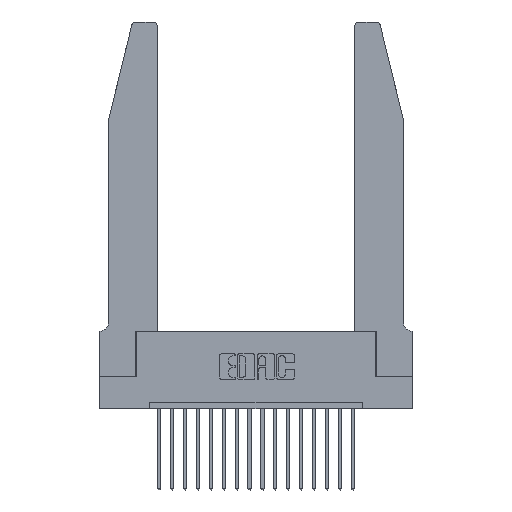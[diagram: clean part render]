
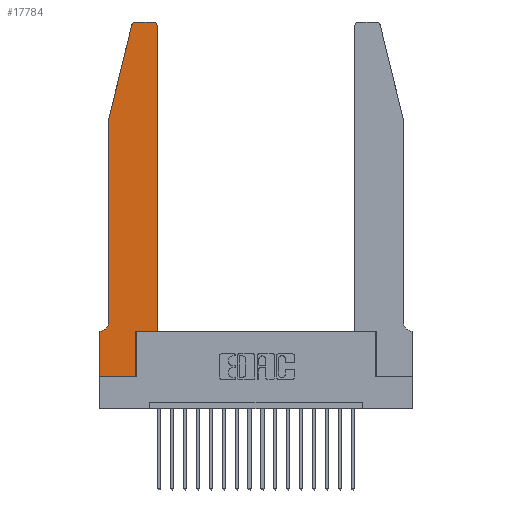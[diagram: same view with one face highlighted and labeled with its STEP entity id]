
A CAD part, top view. The second image highlights one B-rep face of the part: STEP entity #17784.
In plain terms, the highlighted planar face has unit normal (0, 0, 1).
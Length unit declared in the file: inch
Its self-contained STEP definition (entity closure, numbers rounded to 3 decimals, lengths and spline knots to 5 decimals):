
#45 = CIRCLE ( 'NONE', #5649, 0.07 ) ;
#159 = ORIENTED_EDGE ( 'NONE', *, *, #10974, .T. ) ;
#170 = VECTOR ( 'NONE', #8607, 39.37008 ) ;
#180 = ORIENTED_EDGE ( 'NONE', *, *, #13950, .T. ) ;
#245 = CIRCLE ( 'NONE', #19819, 0.03 ) ;
#307 = VECTOR ( 'NONE', #19889, 39.37008 ) ;
#816 = LINE ( 'NONE', #15132, #307 ) ;
#843 = CARTESIAN_POINT ( 'NONE',  ( 0., 0., 0.37 ) ) ;
#1480 = CARTESIAN_POINT ( 'NONE',  ( 0., 0.35, 0.37 ) ) ;
#1695 = DIRECTION ( 'NONE',  ( 1., 0., 0. ) ) ;
#1891 = EDGE_CURVE ( 'NONE', #12858, #2792, #12460, .T. ) ;
#2074 = ORIENTED_EDGE ( 'NONE', *, *, #19408, .T. ) ;
#2139 = ORIENTED_EDGE ( 'NONE', *, *, #1891, .T. ) ;
#2157 = VERTEX_POINT ( 'NONE', #17885 ) ;
#2242 = CARTESIAN_POINT ( 'NONE',  ( 0.0755, 0.42, 0.37 ) ) ;
#2270 = ORIENTED_EDGE ( 'NONE', *, *, #5480, .T. ) ;
#2278 = ORIENTED_EDGE ( 'NONE', *, *, #17199, .T. ) ;
#2341 = VERTEX_POINT ( 'NONE', #13938 ) ;
#2727 = VERTEX_POINT ( 'NONE', #8370 ) ;
#2756 = DIRECTION ( 'NONE',  ( 1., 0., 0. ) ) ;
#2769 = VERTEX_POINT ( 'NONE', #18088 ) ;
#2771 = VERTEX_POINT ( 'NONE', #8446 ) ;
#2792 = VERTEX_POINT ( 'NONE', #16397 ) ;
#3001 = CARTESIAN_POINT ( 'NONE',  ( 0.4505, 0.35, 0.37 ) ) ;
#3121 = CARTESIAN_POINT ( 'NONE',  ( 0.4205, 2.72, 0.37 ) ) ;
#3135 = ORIENTED_EDGE ( 'NONE', *, *, #17731, .T. ) ;
#3656 = EDGE_CURVE ( 'NONE', #15645, #12858, #9179, .T. ) ;
#3837 = DIRECTION ( 'NONE',  ( 1., 0., 0. ) ) ;
#4051 = VECTOR ( 'NONE', #12001, 39.37008 ) ;
#4215 = VECTOR ( 'NONE', #16159, 39.37008 ) ;
#4398 = EDGE_CURVE ( 'NONE', #2341, #15154, #12325, .T. ) ;
#4415 = DIRECTION ( 'NONE',  ( 0., 1., 0. ) ) ;
#4730 = CARTESIAN_POINT ( 'NONE',  ( 0., 0.35, 0.37 ) ) ;
#5480 = EDGE_CURVE ( 'NONE', #12224, #2771, #11797, .T. ) ;
#5498 = ORIENTED_EDGE ( 'NONE', *, *, #3656, .T. ) ;
#5649 = AXIS2_PLACEMENT_3D ( 'NONE', #6503, #19062, #11214 ) ;
#5701 = DIRECTION ( 'NONE',  ( 0., -1., 0. ) ) ;
#5798 = CARTESIAN_POINT ( 'NONE',  ( 0.0755, 0.35, 0.37 ) ) ;
#5837 = DIRECTION ( 'NONE',  ( 0., -1., 0. ) ) ;
#6100 = CARTESIAN_POINT ( 'NONE',  ( 0.0755, 2., 0.37 ) ) ;
#6224 = LINE ( 'NONE', #5798, #4051 ) ;
#6336 = DIRECTION ( 'NONE',  ( 0., 0., 1. ) ) ;
#6437 = FACE_OUTER_BOUND ( 'NONE', #14455, .T. ) ;
#6503 = CARTESIAN_POINT ( 'NONE',  ( 0.0055, 0.42, 0.37 ) ) ;
#6614 = CIRCLE ( 'NONE', #17047, 0.03 ) ;
#6685 = ORIENTED_EDGE ( 'NONE', *, *, #12951, .T. ) ;
#7350 = VECTOR ( 'NONE', #5837, 39.37008 ) ;
#7901 = CARTESIAN_POINT ( 'NONE',  ( 0.2865, 0.35, 0.37 ) ) ;
#8370 = CARTESIAN_POINT ( 'NONE',  ( 0.284, 2.75, 0.37 ) ) ;
#8446 = CARTESIAN_POINT ( 'NONE',  ( 0.4505, 0.35, 0.37 ) ) ;
#8607 = DIRECTION ( 'NONE',  ( -1., 0., 0. ) ) ;
#8786 = CARTESIAN_POINT ( 'NONE',  ( 0.4505, 2.72, 0.37 ) ) ;
#8937 = CARTESIAN_POINT ( 'NONE',  ( 0.4505, 0.35, 0.37 ) ) ;
#9179 = LINE ( 'NONE', #18357, #11635 ) ;
#9505 = CARTESIAN_POINT ( 'NONE',  ( 0.0755, 2., 0.37 ) ) ;
#9609 = VERTEX_POINT ( 'NONE', #8786 ) ;
#10771 = VECTOR ( 'NONE', #3837, 39.37008 ) ;
#10910 = LINE ( 'NONE', #8937, #13366 ) ;
#10974 = EDGE_CURVE ( 'NONE', #20110, #2769, #45, .T. ) ;
#11050 = CARTESIAN_POINT ( 'NONE',  ( 0.284, 2.72, 0.37 ) ) ;
#11214 = DIRECTION ( 'NONE',  ( -1., 0., 0. ) ) ;
#11635 = VECTOR ( 'NONE', #5701, 39.37008 ) ;
#11797 = LINE ( 'NONE', #3001, #4215 ) ;
#11861 = AXIS2_PLACEMENT_3D ( 'NONE', #4730, #12433, #2756 ) ;
#11885 = CARTESIAN_POINT ( 'NONE',  ( 0., 0., 0.37 ) ) ;
#12001 = DIRECTION ( 'NONE',  ( -1., 0., 0. ) ) ;
#12224 = VERTEX_POINT ( 'NONE', #7901 ) ;
#12325 = LINE ( 'NONE', #6100, #14036 ) ;
#12366 = DIRECTION ( 'NONE',  ( -0.239, -0.971, 0. ) ) ;
#12433 = DIRECTION ( 'NONE',  ( 0., 0., 1. ) ) ;
#12460 = LINE ( 'NONE', #11885, #10771 ) ;
#12858 = VERTEX_POINT ( 'NONE', #843 ) ;
#12951 = EDGE_CURVE ( 'NONE', #15154, #20110, #13453, .T. ) ;
#13366 = VECTOR ( 'NONE', #4415, 39.37008 ) ;
#13453 = LINE ( 'NONE', #19884, #7350 ) ;
#13659 = ORIENTED_EDGE ( 'NONE', *, *, #19331, .T. ) ;
#13938 = CARTESIAN_POINT ( 'NONE',  ( 0.25487, 2.72718, 0.37 ) ) ;
#13950 = EDGE_CURVE ( 'NONE', #2157, #2727, #17122, .T. ) ;
#14036 = VECTOR ( 'NONE', #12366, 39.37008 ) ;
#14455 = EDGE_LOOP ( 'NONE', ( #180, #13659, #19462, #6685, #159, #2278, #5498, #2139, #3135, #2270, #19926, #2074 ) ) ;
#14808 = CARTESIAN_POINT ( 'NONE',  ( 0.2605, 2.75, 0.37 ) ) ;
#15132 = CARTESIAN_POINT ( 'NONE',  ( 0.2865, 0.35, 0.37 ) ) ;
#15154 = VERTEX_POINT ( 'NONE', #9505 ) ;
#15645 = VERTEX_POINT ( 'NONE', #1480 ) ;
#15932 = PLANE ( 'NONE',  #11861 ) ;
#16128 = EDGE_CURVE ( 'NONE', #2771, #9609, #10910, .T. ) ;
#16159 = DIRECTION ( 'NONE',  ( 1., 0., 0. ) ) ;
#16397 = CARTESIAN_POINT ( 'NONE',  ( 0.2865, 0., 0.37 ) ) ;
#17047 = AXIS2_PLACEMENT_3D ( 'NONE', #11050, #6336, #1695 ) ;
#17122 = LINE ( 'NONE', #14808, #170 ) ;
#17199 = EDGE_CURVE ( 'NONE', #2769, #15645, #6224, .T. ) ;
#17393 = DIRECTION ( 'NONE',  ( 1., 0., 0. ) ) ;
#17731 = EDGE_CURVE ( 'NONE', #2792, #12224, #816, .T. ) ;
#17784 = ADVANCED_FACE ( 'NONE', ( #6437 ), #15932, .T. ) ;
#17885 = CARTESIAN_POINT ( 'NONE',  ( 0.4205, 2.75, 0.37 ) ) ;
#18088 = CARTESIAN_POINT ( 'NONE',  ( 0.0055, 0.35, 0.37 ) ) ;
#18357 = CARTESIAN_POINT ( 'NONE',  ( 0., 0., 0.37 ) ) ;
#18752 = DIRECTION ( 'NONE',  ( 0., 0., 1. ) ) ;
#19062 = DIRECTION ( 'NONE',  ( 0., 0., -1. ) ) ;
#19331 = EDGE_CURVE ( 'NONE', #2727, #2341, #6614, .T. ) ;
#19408 = EDGE_CURVE ( 'NONE', #9609, #2157, #245, .T. ) ;
#19462 = ORIENTED_EDGE ( 'NONE', *, *, #4398, .T. ) ;
#19819 = AXIS2_PLACEMENT_3D ( 'NONE', #3121, #18752, #17393 ) ;
#19884 = CARTESIAN_POINT ( 'NONE',  ( 0.0755, 2., 0.37 ) ) ;
#19889 = DIRECTION ( 'NONE',  ( 0., 1., 0. ) ) ;
#19926 = ORIENTED_EDGE ( 'NONE', *, *, #16128, .T. ) ;
#20110 = VERTEX_POINT ( 'NONE', #2242 ) ;
